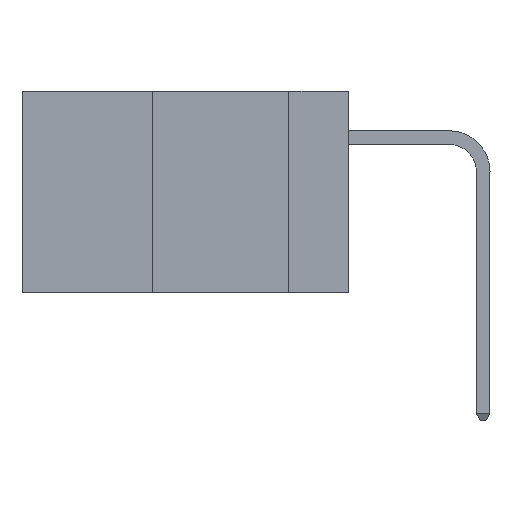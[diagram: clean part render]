
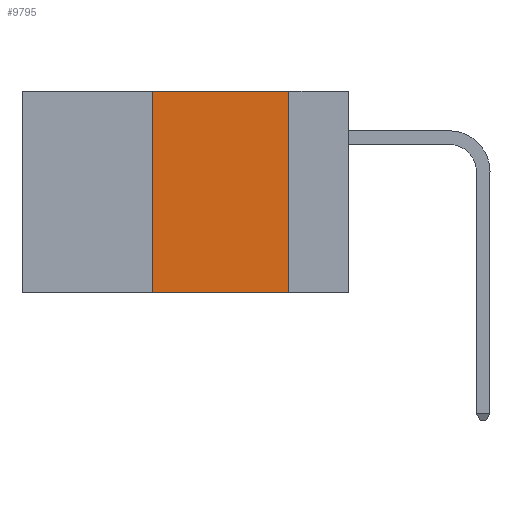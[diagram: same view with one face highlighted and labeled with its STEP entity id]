
A CAD part, left-side view. The second image highlights one B-rep face of the part: STEP entity #9795.
In plain terms, the highlighted planar face has unit normal (-1, 0, 0).
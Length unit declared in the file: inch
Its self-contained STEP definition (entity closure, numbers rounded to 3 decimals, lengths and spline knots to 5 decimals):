
#791 = DIRECTION ( 'NONE',  ( 0., 0., -1. ) ) ;
#1316 = EDGE_LOOP ( 'NONE', ( #3062, #32587, #32241, #21161 ) ) ;
#1950 = LINE ( 'NONE', #27539, #29415 ) ;
#2243 = VECTOR ( 'NONE', #15696, 39.37008 ) ;
#3062 = ORIENTED_EDGE ( 'NONE', *, *, #30105, .F. ) ;
#3795 = VECTOR ( 'NONE', #11605, 39.37008 ) ;
#6509 = DIRECTION ( 'NONE',  ( 1., 0., 0. ) ) ;
#8432 = VERTEX_POINT ( 'NONE', #10902 ) ;
#9795 = ADVANCED_FACE ( 'NONE', ( #36364 ), #18049, .F. ) ;
#10017 = CARTESIAN_POINT ( 'NONE',  ( 0., 0.6, 0. ) ) ;
#10902 = CARTESIAN_POINT ( 'NONE',  ( 0., 0.11, 0. ) ) ;
#11605 = DIRECTION ( 'NONE',  ( 0., -1., 0. ) ) ;
#12186 = VERTEX_POINT ( 'NONE', #20584 ) ;
#13277 = CARTESIAN_POINT ( 'NONE',  ( 0., 0.11, -0.37 ) ) ;
#14717 = CARTESIAN_POINT ( 'NONE',  ( 0., 0.6, -0.37 ) ) ;
#15696 = DIRECTION ( 'NONE',  ( 0., -1., 0. ) ) ;
#18049 = PLANE ( 'NONE',  #26459 ) ;
#19033 = EDGE_CURVE ( 'NONE', #12186, #22385, #19989, .T. ) ;
#19597 = LINE ( 'NONE', #29567, #33269 ) ;
#19989 = LINE ( 'NONE', #14717, #3795 ) ;
#20584 = CARTESIAN_POINT ( 'NONE',  ( 0., 0.36, -0.37 ) ) ;
#20904 = EDGE_CURVE ( 'NONE', #12186, #36239, #19597, .T. ) ;
#21161 = ORIENTED_EDGE ( 'NONE', *, *, #19033, .T. ) ;
#22385 = VERTEX_POINT ( 'NONE', #13277 ) ;
#24913 = EDGE_CURVE ( 'NONE', #36239, #8432, #33040, .T. ) ;
#26459 = AXIS2_PLACEMENT_3D ( 'NONE', #31755, #6509, #791 ) ;
#27539 = CARTESIAN_POINT ( 'NONE',  ( 0., 0.11, 0. ) ) ;
#29415 = VECTOR ( 'NONE', #30231, 39.37008 ) ;
#29567 = CARTESIAN_POINT ( 'NONE',  ( 0., 0.36, 0. ) ) ;
#30105 = EDGE_CURVE ( 'NONE', #8432, #22385, #1950, .T. ) ;
#30231 = DIRECTION ( 'NONE',  ( 0., 0., -1. ) ) ;
#31755 = CARTESIAN_POINT ( 'NONE',  ( 0., 0.6, 0. ) ) ;
#32222 = DIRECTION ( 'NONE',  ( 0., 0., 1. ) ) ;
#32241 = ORIENTED_EDGE ( 'NONE', *, *, #20904, .F. ) ;
#32587 = ORIENTED_EDGE ( 'NONE', *, *, #24913, .F. ) ;
#33040 = LINE ( 'NONE', #10017, #2243 ) ;
#33269 = VECTOR ( 'NONE', #32222, 39.37008 ) ;
#33462 = CARTESIAN_POINT ( 'NONE',  ( 0., 0.36, 0. ) ) ;
#36239 = VERTEX_POINT ( 'NONE', #33462 ) ;
#36364 = FACE_OUTER_BOUND ( 'NONE', #1316, .T. ) ;
